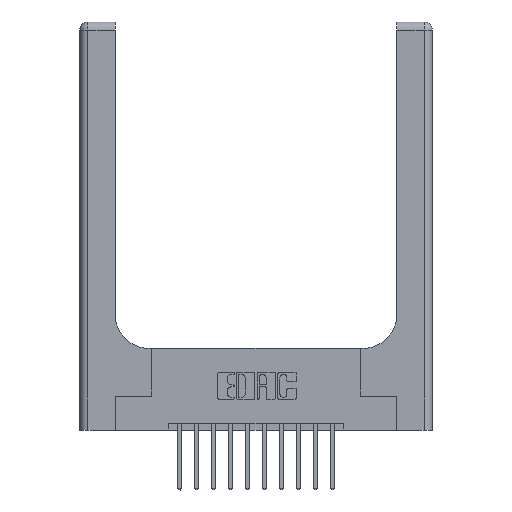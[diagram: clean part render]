
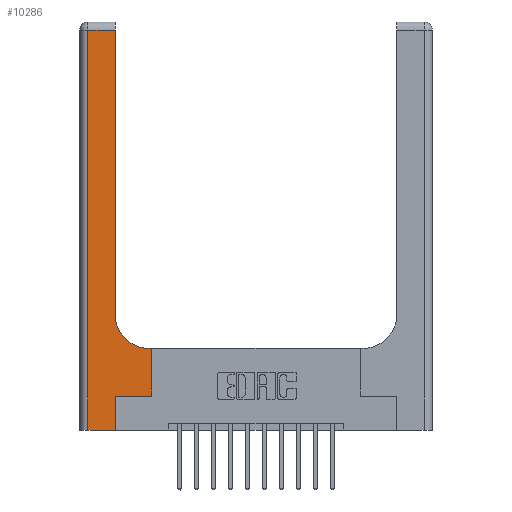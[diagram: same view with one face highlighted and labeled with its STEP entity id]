
A CAD part, top view. The second image highlights one B-rep face of the part: STEP entity #10286.
In plain terms, the highlighted planar face has unit normal (0, 0, 1).
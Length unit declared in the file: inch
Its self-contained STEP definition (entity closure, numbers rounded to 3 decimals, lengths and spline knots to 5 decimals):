
#214 = DIRECTION ( 'NONE',  ( 1., 0., 0. ) ) ;
#314 = LINE ( 'NONE', #7122, #11978 ) ;
#1203 = DIRECTION ( 'NONE',  ( -1., 0., 0. ) ) ;
#1309 = CARTESIAN_POINT ( 'NONE',  ( 0.51, 0.6, 0.37 ) ) ;
#1365 = PLANE ( 'NONE',  #11970 ) ;
#1452 = DIRECTION ( 'NONE',  ( 0., 1., 0. ) ) ;
#1468 = DIRECTION ( 'NONE',  ( -1., 0., 0. ) ) ;
#1968 = VECTOR ( 'NONE', #15523, 39.37008 ) ;
#2007 = CARTESIAN_POINT ( 'NONE',  ( 0.528, 0.25, 0.37 ) ) ;
#2170 = CARTESIAN_POINT ( 'NONE',  ( 0.26, 0.85, 0.37 ) ) ;
#2386 = CARTESIAN_POINT ( 'NONE',  ( 0.06, 2.94, 0.37 ) ) ;
#2626 = ORIENTED_EDGE ( 'NONE', *, *, #5637, .T. ) ;
#2647 = FACE_OUTER_BOUND ( 'NONE', #15197, .T. ) ;
#2812 = LINE ( 'NONE', #9641, #4948 ) ;
#2825 = EDGE_CURVE ( 'NONE', #3950, #4238, #9576, .T. ) ;
#2902 = CARTESIAN_POINT ( 'NONE',  ( 0.528, 0.6, 0.37 ) ) ;
#3161 = VERTEX_POINT ( 'NONE', #1309 ) ;
#3389 = LINE ( 'NONE', #8779, #10010 ) ;
#3754 = ORIENTED_EDGE ( 'NONE', *, *, #4031, .T. ) ;
#3767 = DIRECTION ( 'NONE',  ( 1., 0., 0. ) ) ;
#3950 = VERTEX_POINT ( 'NONE', #15239 ) ;
#4031 = EDGE_CURVE ( 'NONE', #4238, #14593, #10898, .T. ) ;
#4238 = VERTEX_POINT ( 'NONE', #2386 ) ;
#4616 = DIRECTION ( 'NONE',  ( 0., 1., 0. ) ) ;
#4948 = VECTOR ( 'NONE', #4616, 39.37008 ) ;
#5021 = VECTOR ( 'NONE', #11645, 39.37008 ) ;
#5179 = CARTESIAN_POINT ( 'NONE',  ( 0.528, 0.25, 0.37 ) ) ;
#5513 = EDGE_CURVE ( 'NONE', #12162, #3161, #8897, .T. ) ;
#5637 = EDGE_CURVE ( 'NONE', #10043, #12162, #13752, .T. ) ;
#5830 = AXIS2_PLACEMENT_3D ( 'NONE', #9989, #6219, #11247 ) ;
#5990 = VECTOR ( 'NONE', #1203, 39.37008 ) ;
#6219 = DIRECTION ( 'NONE',  ( 0., 0., -1. ) ) ;
#6848 = CARTESIAN_POINT ( 'NONE',  ( 0., 2.94, 0.37 ) ) ;
#7122 = CARTESIAN_POINT ( 'NONE',  ( 0.265, 0., 0.37 ) ) ;
#7317 = CARTESIAN_POINT ( 'NONE',  ( 0.265, 0.25, 0.37 ) ) ;
#7551 = DIRECTION ( 'NONE',  ( 0., 0., -1. ) ) ;
#8183 = ORIENTED_EDGE ( 'NONE', *, *, #15770, .T. ) ;
#8630 = VERTEX_POINT ( 'NONE', #2170 ) ;
#8779 = CARTESIAN_POINT ( 'NONE',  ( 0., 0., 0.37 ) ) ;
#8841 = ORIENTED_EDGE ( 'NONE', *, *, #11338, .T. ) ;
#8897 = LINE ( 'NONE', #13662, #5990 ) ;
#9471 = VECTOR ( 'NONE', #3767, 39.37008 ) ;
#9576 = LINE ( 'NONE', #6848, #1968 ) ;
#9635 = DIRECTION ( 'NONE',  ( 0., 1., 0. ) ) ;
#9641 = CARTESIAN_POINT ( 'NONE',  ( 0.26, 3., 0.37 ) ) ;
#9668 = LINE ( 'NONE', #9992, #9471 ) ;
#9890 = VECTOR ( 'NONE', #1452, 39.37008 ) ;
#9989 = CARTESIAN_POINT ( 'NONE',  ( 0.51, 0.85, 0.37 ) ) ;
#9992 = CARTESIAN_POINT ( 'NONE',  ( 0.265, 0.25, 0.37 ) ) ;
#10010 = VECTOR ( 'NONE', #214, 39.37008 ) ;
#10043 = VERTEX_POINT ( 'NONE', #2007 ) ;
#10286 = ADVANCED_FACE ( 'NONE', ( #2647 ), #1365, .F. ) ;
#10697 = ORIENTED_EDGE ( 'NONE', *, *, #2825, .T. ) ;
#10898 = LINE ( 'NONE', #15298, #5021 ) ;
#11247 = DIRECTION ( 'NONE',  ( 1., 0., 0. ) ) ;
#11338 = EDGE_CURVE ( 'NONE', #8630, #3950, #2812, .T. ) ;
#11645 = DIRECTION ( 'NONE',  ( 0., -1., 0. ) ) ;
#11944 = ORIENTED_EDGE ( 'NONE', *, *, #15676, .T. ) ;
#11970 = AXIS2_PLACEMENT_3D ( 'NONE', #12591, #7551, #1468 ) ;
#11978 = VECTOR ( 'NONE', #9635, 39.37008 ) ;
#12017 = EDGE_CURVE ( 'NONE', #14593, #14186, #3389, .T. ) ;
#12162 = VERTEX_POINT ( 'NONE', #2902 ) ;
#12591 = CARTESIAN_POINT ( 'NONE',  ( 0., 3., 0.37 ) ) ;
#13233 = CIRCLE ( 'NONE', #5830, 0.25 ) ;
#13662 = CARTESIAN_POINT ( 'NONE',  ( 0.26, 0.6, 0.37 ) ) ;
#13670 = ORIENTED_EDGE ( 'NONE', *, *, #5513, .T. ) ;
#13752 = LINE ( 'NONE', #5179, #9890 ) ;
#13793 = EDGE_CURVE ( 'NONE', #3161, #8630, #13233, .T. ) ;
#13858 = VERTEX_POINT ( 'NONE', #7317 ) ;
#14186 = VERTEX_POINT ( 'NONE', #15699 ) ;
#14369 = ORIENTED_EDGE ( 'NONE', *, *, #13793, .T. ) ;
#14593 = VERTEX_POINT ( 'NONE', #15079 ) ;
#15079 = CARTESIAN_POINT ( 'NONE',  ( 0.06, 0., 0.37 ) ) ;
#15197 = EDGE_LOOP ( 'NONE', ( #8841, #10697, #3754, #15513, #8183, #11944, #2626, #13670, #14369 ) ) ;
#15239 = CARTESIAN_POINT ( 'NONE',  ( 0.26, 2.94, 0.37 ) ) ;
#15298 = CARTESIAN_POINT ( 'NONE',  ( 0.06, 3., 0.37 ) ) ;
#15513 = ORIENTED_EDGE ( 'NONE', *, *, #12017, .T. ) ;
#15523 = DIRECTION ( 'NONE',  ( -1., 0., 0. ) ) ;
#15676 = EDGE_CURVE ( 'NONE', #13858, #10043, #9668, .T. ) ;
#15699 = CARTESIAN_POINT ( 'NONE',  ( 0.265, 0., 0.37 ) ) ;
#15770 = EDGE_CURVE ( 'NONE', #14186, #13858, #314, .T. ) ;
